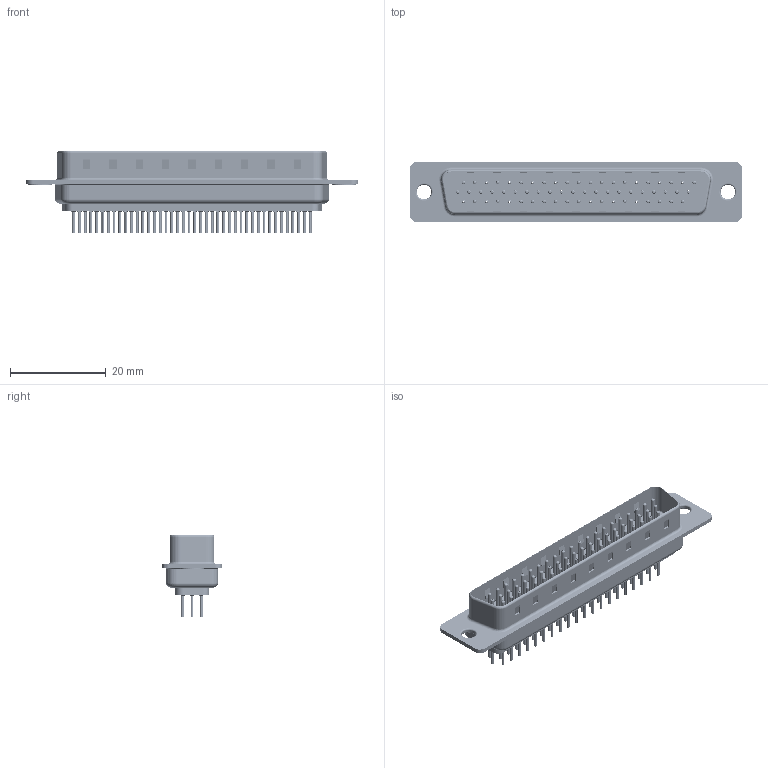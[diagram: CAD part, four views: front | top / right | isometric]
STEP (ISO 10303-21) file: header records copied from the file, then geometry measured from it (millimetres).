
FILE_DESCRIPTION (( 'STEP AP203' ), '1' );
FILE_NAME ('637-062-630-061.STEP', '2020-07-18T04:32:58', ( '' ), ( '' ), 'SwSTEP 2.0', 'SolidWorks 2020', '' );
FILE_SCHEMA (( 'CONFIG_CONTROL_DESIGN' ));
Length unit declared in the file: millimetre
Products named in the file (8): 637 Shell Rear_62 Contacts; 637 Shell Front_62 Contacts; 637-062-630-061; 637 Thru Hole Rivet; 637 Contact Row 1_30; 637 Contact Row 3_30; 637 Housing_62 Contacts; 637 Contact Row 2_30
Assembly tree (67 placements, depth 2):
  637-062-630-061
    637 Housing_62 Contacts
    637 Shell Front_62 Contacts
    637 Shell Rear_62 Contacts
    637 Contact Row 1_30  x21
    637 Contact Row 2_30  x21
    637 Contact Row 3_30  x20
    637 Thru Hole Rivet  x2
Bounding box: 69.4 x 12.6 x 17.25 mm (x, y, z)
Volume: 3610.1 mm3; surface area: 13476.4 mm2
Topology: 67 solids, 67 shells, 6586 faces, 17405 edges, 10716 vertices
Faces by surface type: cylinder 2419, torus 1856, plane 1691, cone 620
Entity records: 37490 total; most frequent: CARTESIAN_POINT 6622, DIRECTION 6484, ORIENTED_EDGE 5536, EDGE_CURVE 2768, AXIS2_PLACEMENT_3D 2625, VERTEX_POINT 1777, EDGE_LOOP 1445, CIRCLE 1417
